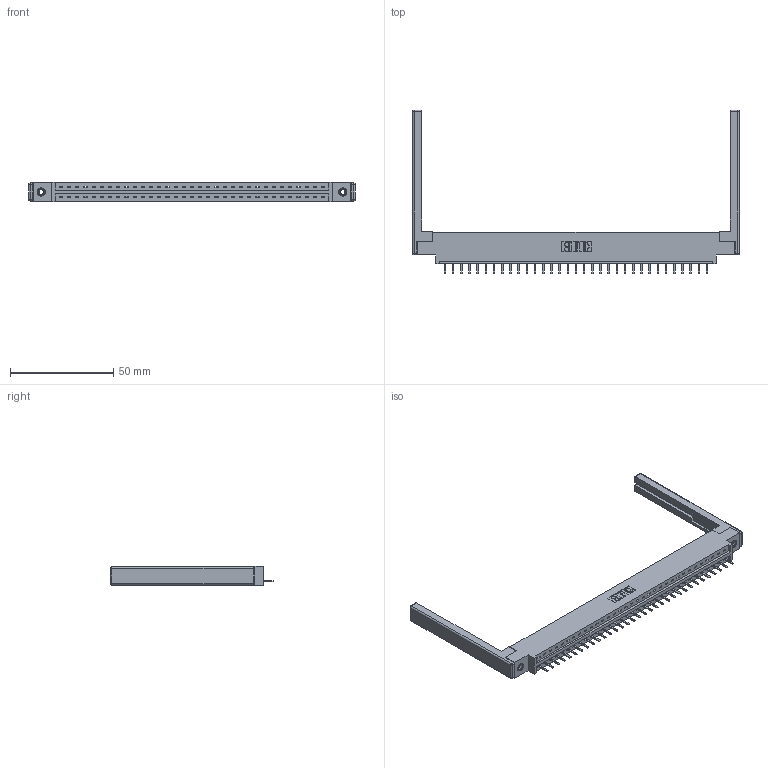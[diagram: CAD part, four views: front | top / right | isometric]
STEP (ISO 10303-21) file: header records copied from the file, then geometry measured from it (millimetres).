
FILE_DESCRIPTION (( 'STEP AP203' ), '1' );
FILE_NAME ('387-033-520-668.STEP', '2019-10-03T21:30:49', ( '' ), ( '' ), 'SwSTEP 2.0', 'SolidWorks 2016', '' );
FILE_SCHEMA (( 'CONFIG_CONTROL_DESIGN' ));
Length unit declared in the file: inch
Products named in the file (5): 345-250-001_345-250-001-102; 387-033-520-668; 307-220-068; 337 Part_0.170 Offset - 0.156 Dia-TI; 345-292-001_345-293-120
Assembly tree (38 placements, depth 2):
  387-033-520-668
    337 Part_0.170 Offset - 0.156 Dia-TI
    345-292-001_345-293-120  x33
    345-250-001_345-250-001-102  x2
    307-220-068  x2
Bounding box: 158.19 x 79.08 x 9.4 mm (x, y, z)
Volume: 20507.5 mm3; surface area: 20451.2 mm2
Topology: 38 solids, 38 shells, 2450 faces, 7181 edges, 4678 vertices
Faces by surface type: plane 1746, cylinder 680, cone 12, sphere 8, torus 4
Entity records: 28700 total; most frequent: CARTESIAN_POINT 4966, ORIENTED_EDGE 4912, DIRECTION 4260, EDGE_CURVE 2456, LINE 2274, VECTOR 2274, VERTEX_POINT 1626, AXIS2_PLACEMENT_3D 993
